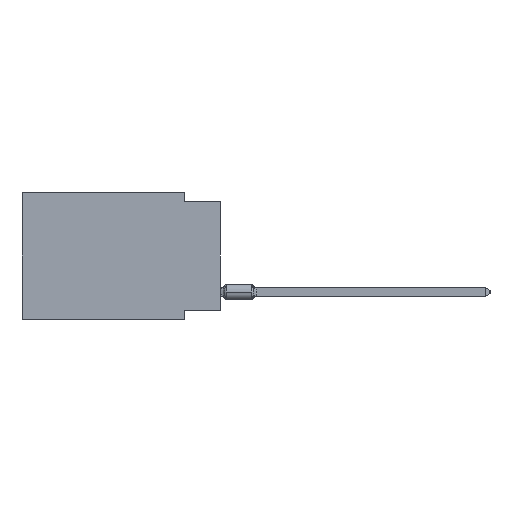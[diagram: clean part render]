
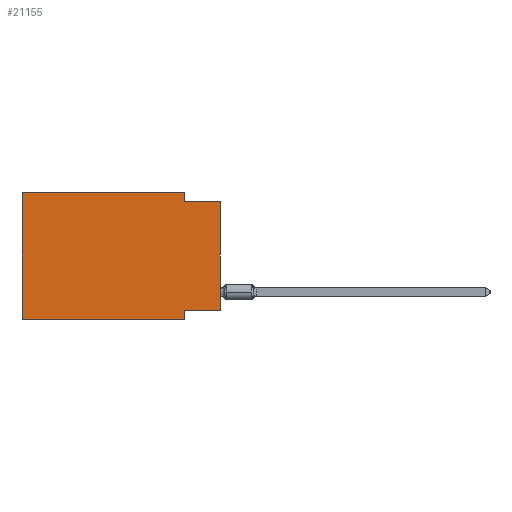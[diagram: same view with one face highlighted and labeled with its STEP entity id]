
A CAD part, left-side view. The second image highlights one B-rep face of the part: STEP entity #21155.
In plain terms, the highlighted planar face has unit normal (-1, 0, 0).
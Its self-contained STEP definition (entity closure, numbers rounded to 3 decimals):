
#1767 = LINE ( 'NONE', #37974, #29427 ) ;
#2524 = EDGE_CURVE ( 'NONE', #7206, #30410, #39899, .T. ) ;
#2531 = CARTESIAN_POINT ( 'NONE',  ( 0., 13.97, 0. ) ) ;
#2960 = CARTESIAN_POINT ( 'NONE',  ( 0., 2.54, -8.89 ) ) ;
#3414 = ORIENTED_EDGE ( 'NONE', *, *, #46909, .F. ) ;
#3684 = VECTOR ( 'NONE', #38726, 1000. ) ;
#4261 = VERTEX_POINT ( 'NONE', #2960 ) ;
#6695 = DIRECTION ( 'NONE',  ( 0., -1., 0. ) ) ;
#7206 = VERTEX_POINT ( 'NONE', #16661 ) ;
#7950 = LINE ( 'NONE', #10819, #28813 ) ;
#8665 = CARTESIAN_POINT ( 'NONE',  ( 0., 13.97, 0. ) ) ;
#9596 = CARTESIAN_POINT ( 'NONE',  ( 0., 0., -0.635 ) ) ;
#10819 = CARTESIAN_POINT ( 'NONE',  ( 0., 2.54, -8.89 ) ) ;
#11088 = ORIENTED_EDGE ( 'NONE', *, *, #2524, .F. ) ;
#11107 = CARTESIAN_POINT ( 'NONE',  ( 0., 13.97, 0. ) ) ;
#11393 = CARTESIAN_POINT ( 'NONE',  ( 0., 0., -8.255 ) ) ;
#13103 = LINE ( 'NONE', #2531, #29724 ) ;
#13166 = CARTESIAN_POINT ( 'NONE',  ( 0., 2.54, -8.255 ) ) ;
#13174 = EDGE_LOOP ( 'NONE', ( #36796, #19725, #16720, #3414, #11088, #23904, #20075, #16898 ) ) ;
#15705 = VERTEX_POINT ( 'NONE', #11393 ) ;
#16661 = CARTESIAN_POINT ( 'NONE',  ( 0., 13.97, -8.89 ) ) ;
#16720 = ORIENTED_EDGE ( 'NONE', *, *, #46974, .F. ) ;
#16898 = ORIENTED_EDGE ( 'NONE', *, *, #33434, .F. ) ;
#16913 = DIRECTION ( 'NONE',  ( 0., -1., 0. ) ) ;
#16950 = CARTESIAN_POINT ( 'NONE',  ( 0., 2.54, 0. ) ) ;
#17217 = LINE ( 'NONE', #17441, #28471 ) ;
#17441 = CARTESIAN_POINT ( 'NONE',  ( 0., 0., -8.255 ) ) ;
#17512 = VECTOR ( 'NONE', #33750, 1000. ) ;
#17724 = VERTEX_POINT ( 'NONE', #42838 ) ;
#17756 = LINE ( 'NONE', #9596, #29242 ) ;
#18067 = EDGE_CURVE ( 'NONE', #7206, #4261, #1767, .T. ) ;
#18239 = PLANE ( 'NONE',  #36634 ) ;
#19725 = ORIENTED_EDGE ( 'NONE', *, *, #29256, .F. ) ;
#20075 = ORIENTED_EDGE ( 'NONE', *, *, #30812, .F. ) ;
#21155 = ADVANCED_FACE ( 'NONE', ( #39799 ), #18239, .F. ) ;
#21207 = EDGE_CURVE ( 'NONE', #15705, #41869, #36426, .T. ) ;
#21354 = DIRECTION ( 'NONE',  ( 0., 0., -1. ) ) ;
#23904 = ORIENTED_EDGE ( 'NONE', *, *, #18067, .T. ) ;
#28471 = VECTOR ( 'NONE', #35639, 1000. ) ;
#28813 = VECTOR ( 'NONE', #44143, 1000. ) ;
#29242 = VECTOR ( 'NONE', #6695, 1000. ) ;
#29256 = EDGE_CURVE ( 'NONE', #47377, #41869, #17756, .T. ) ;
#29427 = VECTOR ( 'NONE', #16913, 1000. ) ;
#29476 = CARTESIAN_POINT ( 'NONE',  ( 0., 13.97, 0. ) ) ;
#29724 = VECTOR ( 'NONE', #46663, 1000. ) ;
#29747 = VERTEX_POINT ( 'NONE', #13166 ) ;
#30410 = VERTEX_POINT ( 'NONE', #8665 ) ;
#30812 = EDGE_CURVE ( 'NONE', #29747, #4261, #7950, .T. ) ;
#32812 = CARTESIAN_POINT ( 'NONE',  ( 0., 0., 0. ) ) ;
#33434 = EDGE_CURVE ( 'NONE', #15705, #29747, #17217, .T. ) ;
#33750 = DIRECTION ( 'NONE',  ( 0., 0., 1. ) ) ;
#35133 = LINE ( 'NONE', #16950, #3684 ) ;
#35639 = DIRECTION ( 'NONE',  ( 0., 1., 0. ) ) ;
#36239 = CARTESIAN_POINT ( 'NONE',  ( 0., 2.54, -0.635 ) ) ;
#36426 = LINE ( 'NONE', #32812, #17512 ) ;
#36634 = AXIS2_PLACEMENT_3D ( 'NONE', #29476, #44117, #21354 ) ;
#36796 = ORIENTED_EDGE ( 'NONE', *, *, #21207, .T. ) ;
#37512 = VECTOR ( 'NONE', #47349, 1000. ) ;
#37974 = CARTESIAN_POINT ( 'NONE',  ( 0., 13.97, -8.89 ) ) ;
#38726 = DIRECTION ( 'NONE',  ( 0., 0., -1. ) ) ;
#39799 = FACE_OUTER_BOUND ( 'NONE', #13174, .T. ) ;
#39899 = LINE ( 'NONE', #11107, #37512 ) ;
#41869 = VERTEX_POINT ( 'NONE', #43611 ) ;
#42838 = CARTESIAN_POINT ( 'NONE',  ( 0., 2.54, 0. ) ) ;
#43611 = CARTESIAN_POINT ( 'NONE',  ( 0., 0., -0.635 ) ) ;
#44117 = DIRECTION ( 'NONE',  ( 1., 0., 0. ) ) ;
#44143 = DIRECTION ( 'NONE',  ( 0., 0., -1. ) ) ;
#46663 = DIRECTION ( 'NONE',  ( 0., -1., 0. ) ) ;
#46909 = EDGE_CURVE ( 'NONE', #30410, #17724, #13103, .T. ) ;
#46974 = EDGE_CURVE ( 'NONE', #17724, #47377, #35133, .T. ) ;
#47349 = DIRECTION ( 'NONE',  ( 0., 0., 1. ) ) ;
#47377 = VERTEX_POINT ( 'NONE', #36239 ) ;
